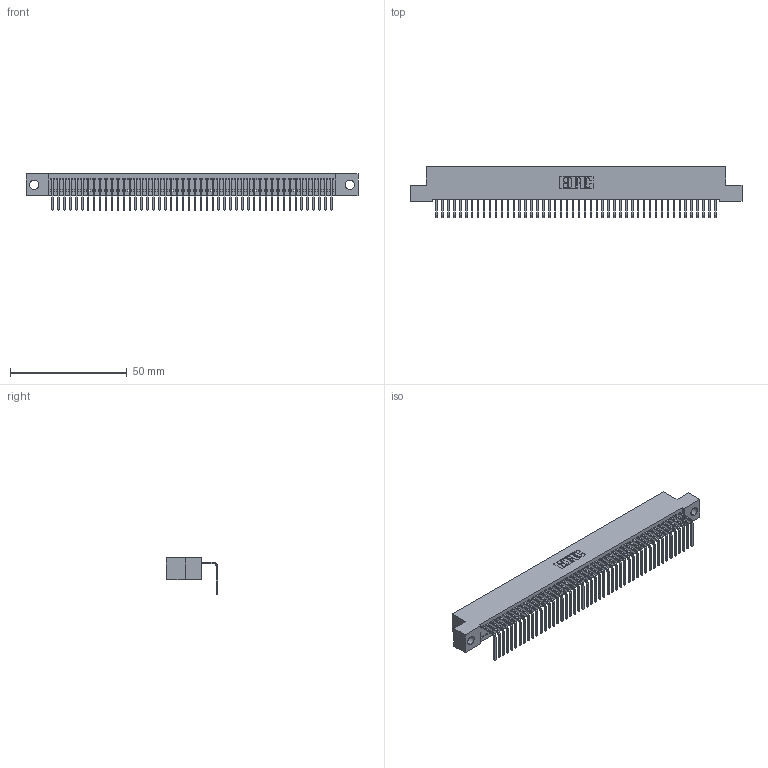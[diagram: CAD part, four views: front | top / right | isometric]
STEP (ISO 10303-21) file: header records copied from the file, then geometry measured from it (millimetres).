
FILE_DESCRIPTION (( 'STEP AP203' ), '1' );
FILE_NAME ('342-048-558-104.STEP', '2018-08-12T18:24:10', ( '' ), ( '' ), 'SwSTEP 2.0', 'SolidWorks 2016', '' );
FILE_SCHEMA (( 'CONFIG_CONTROL_DESIGN' ));
Length unit declared in the file: inch
Products named in the file (3): 342 Part_.156 TH; 345-292-001_558 Tail - 2; 342-048-558-104
Assembly tree (49 placements, depth 2):
  342-048-558-104
    342 Part_.156 TH
    345-292-001_558 Tail - 2  x48
Bounding box: 142.24 x 21.91 x 15.62 mm (x, y, z)
Volume: 12566.6 mm3; surface area: 19292.6 mm2
Topology: 49 solids, 49 shells, 2990 faces, 9035 edges, 5958 vertices
Faces by surface type: plane 2178, cylinder 812
Entity records: 28523 total; most frequent: CARTESIAN_POINT 4926, ORIENTED_EDGE 4910, DIRECTION 4143, EDGE_CURVE 2455, VECTOR 2327, LINE 2327, VERTEX_POINT 1634, AXIS2_PLACEMENT_3D 908
